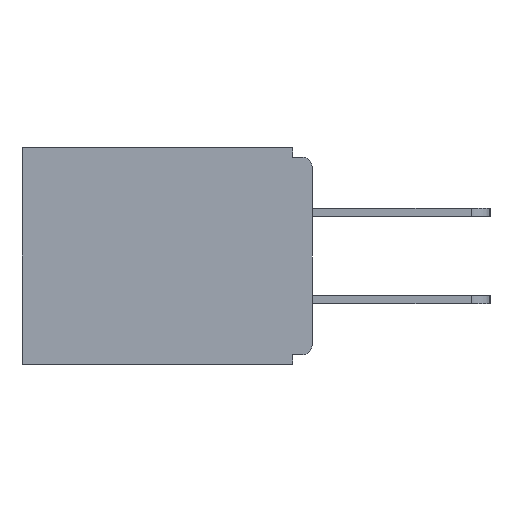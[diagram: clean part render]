
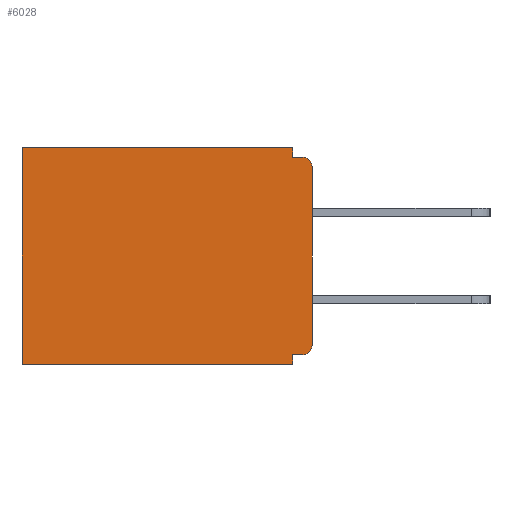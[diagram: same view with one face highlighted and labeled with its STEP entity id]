
A CAD part, left-side view. The second image highlights one B-rep face of the part: STEP entity #6028.
In plain terms, the highlighted planar face has unit normal (-1, 0, 0).
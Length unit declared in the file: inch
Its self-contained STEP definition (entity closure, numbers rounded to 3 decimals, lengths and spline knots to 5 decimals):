
#11 = DIRECTION ( 'NONE',  ( 0., 1., 0. ) ) ;
#64 = FACE_OUTER_BOUND ( 'NONE', #15069, .T. ) ;
#215 = CARTESIAN_POINT ( 'NONE',  ( 0.298, 0., 0. ) ) ;
#602 = CARTESIAN_POINT ( 'NONE',  ( 0.298, 0.46, 0. ) ) ;
#608 = CARTESIAN_POINT ( 'NONE',  ( 0.298, 0.015, -0.03 ) ) ;
#649 = EDGE_CURVE ( 'NONE', #14094, #7322, #11745, .T. ) ;
#720 = VERTEX_POINT ( 'NONE', #4640 ) ;
#843 = CARTESIAN_POINT ( 'NONE',  ( 0.298, 0.031, -0.328 ) ) ;
#852 = EDGE_CURVE ( 'NONE', #11804, #15190, #6631, .T. ) ;
#913 = CIRCLE ( 'NONE', #3900, 0.015 ) ;
#1393 = CARTESIAN_POINT ( 'NONE',  ( 0.298, 0., -0.328 ) ) ;
#1752 = DIRECTION ( 'NONE',  ( 0., 0., -1. ) ) ;
#1772 = EDGE_CURVE ( 'NONE', #8749, #11788, #9150, .T. ) ;
#1929 = EDGE_CURVE ( 'NONE', #8749, #8089, #913, .T. ) ;
#2043 = CARTESIAN_POINT ( 'NONE',  ( 0.298, 0., -0.03 ) ) ;
#2549 = VECTOR ( 'NONE', #9634, 39.37008 ) ;
#2890 = DIRECTION ( 'NONE',  ( -1., 0., 0. ) ) ;
#3313 = EDGE_CURVE ( 'NONE', #720, #7322, #11913, .T. ) ;
#3400 = CIRCLE ( 'NONE', #14229, 0.015 ) ;
#3420 = LINE ( 'NONE', #4873, #13512 ) ;
#3453 = VECTOR ( 'NONE', #11, 39.37008 ) ;
#3592 = ORIENTED_EDGE ( 'NONE', *, *, #13378, .F. ) ;
#3638 = CARTESIAN_POINT ( 'NONE',  ( 0.298, 0., 0. ) ) ;
#3900 = AXIS2_PLACEMENT_3D ( 'NONE', #5189, #10061, #6422 ) ;
#3957 = LINE ( 'NONE', #6035, #8710 ) ;
#4184 = DIRECTION ( 'NONE',  ( 0., 0., -1. ) ) ;
#4640 = CARTESIAN_POINT ( 'NONE',  ( 0.298, 0.031, -0.343 ) ) ;
#4873 = CARTESIAN_POINT ( 'NONE',  ( 0.298, 0., -0.015 ) ) ;
#4896 = ORIENTED_EDGE ( 'NONE', *, *, #852, .F. ) ;
#4898 = PLANE ( 'NONE',  #9255 ) ;
#5189 = CARTESIAN_POINT ( 'NONE',  ( 0.298, 0.015, -0.313 ) ) ;
#5520 = EDGE_CURVE ( 'NONE', #7684, #11739, #3400, .T. ) ;
#5567 = CARTESIAN_POINT ( 'NONE',  ( 0.298, 0., 0. ) ) ;
#5697 = ORIENTED_EDGE ( 'NONE', *, *, #1772, .F. ) ;
#5848 = ORIENTED_EDGE ( 'NONE', *, *, #5520, .T. ) ;
#6028 = ADVANCED_FACE ( 'NONE', ( #64 ), #4898, .F. ) ;
#6035 = CARTESIAN_POINT ( 'NONE',  ( 0.298, 0.031, -0.343 ) ) ;
#6422 = DIRECTION ( 'NONE',  ( 0., 0., -1. ) ) ;
#6631 = LINE ( 'NONE', #11407, #13027 ) ;
#6673 = EDGE_CURVE ( 'NONE', #11804, #14094, #13453, .T. ) ;
#7056 = VECTOR ( 'NONE', #9586, 39.37008 ) ;
#7313 = CARTESIAN_POINT ( 'NONE',  ( 0.298, 0.031, -0.015 ) ) ;
#7322 = VERTEX_POINT ( 'NONE', #14557 ) ;
#7684 = VERTEX_POINT ( 'NONE', #2043 ) ;
#8089 = VERTEX_POINT ( 'NONE', #11778 ) ;
#8325 = ORIENTED_EDGE ( 'NONE', *, *, #6673, .T. ) ;
#8421 = ORIENTED_EDGE ( 'NONE', *, *, #1929, .T. ) ;
#8512 = DIRECTION ( 'NONE',  ( 0., -1., 0. ) ) ;
#8710 = VECTOR ( 'NONE', #13284, 39.37008 ) ;
#8749 = VERTEX_POINT ( 'NONE', #12000 ) ;
#8943 = VECTOR ( 'NONE', #4184, 39.37008 ) ;
#9150 = LINE ( 'NONE', #1393, #2549 ) ;
#9255 = AXIS2_PLACEMENT_3D ( 'NONE', #215, #14837, #1752 ) ;
#9586 = DIRECTION ( 'NONE',  ( 0., 0., -1. ) ) ;
#9634 = DIRECTION ( 'NONE',  ( 0., 1., 0. ) ) ;
#10061 = DIRECTION ( 'NONE',  ( -1., 0., 0. ) ) ;
#10394 = ORIENTED_EDGE ( 'NONE', *, *, #13157, .F. ) ;
#10799 = CARTESIAN_POINT ( 'NONE',  ( 0.298, 0.015, -0.015 ) ) ;
#11304 = DIRECTION ( 'NONE',  ( 0., 0., -1. ) ) ;
#11407 = CARTESIAN_POINT ( 'NONE',  ( 0.298, 0.031, -0.343 ) ) ;
#11495 = CARTESIAN_POINT ( 'NONE',  ( 0.298, 0.46, 0. ) ) ;
#11739 = VERTEX_POINT ( 'NONE', #10799 ) ;
#11745 = LINE ( 'NONE', #11495, #7056 ) ;
#11769 = LINE ( 'NONE', #5567, #8943 ) ;
#11778 = CARTESIAN_POINT ( 'NONE',  ( 0.298, 0., -0.313 ) ) ;
#11788 = VERTEX_POINT ( 'NONE', #843 ) ;
#11804 = VERTEX_POINT ( 'NONE', #12728 ) ;
#11913 = LINE ( 'NONE', #14531, #3453 ) ;
#12000 = CARTESIAN_POINT ( 'NONE',  ( 0.298, 0.015, -0.328 ) ) ;
#12728 = CARTESIAN_POINT ( 'NONE',  ( 0.298, 0.031, 0. ) ) ;
#13027 = VECTOR ( 'NONE', #11304, 39.37008 ) ;
#13065 = EDGE_CURVE ( 'NONE', #15190, #11739, #3420, .T. ) ;
#13157 = EDGE_CURVE ( 'NONE', #11788, #720, #3957, .T. ) ;
#13201 = DIRECTION ( 'NONE',  ( 0., 1., 0. ) ) ;
#13284 = DIRECTION ( 'NONE',  ( 0., 0., -1. ) ) ;
#13378 = EDGE_CURVE ( 'NONE', #7684, #8089, #11769, .T. ) ;
#13453 = LINE ( 'NONE', #3638, #14580 ) ;
#13512 = VECTOR ( 'NONE', #8512, 39.37008 ) ;
#14074 = ORIENTED_EDGE ( 'NONE', *, *, #649, .T. ) ;
#14094 = VERTEX_POINT ( 'NONE', #602 ) ;
#14229 = AXIS2_PLACEMENT_3D ( 'NONE', #608, #2890, #14731 ) ;
#14531 = CARTESIAN_POINT ( 'NONE',  ( 0.298, 0., -0.343 ) ) ;
#14557 = CARTESIAN_POINT ( 'NONE',  ( 0.298, 0.46, -0.343 ) ) ;
#14580 = VECTOR ( 'NONE', #13201, 39.37008 ) ;
#14731 = DIRECTION ( 'NONE',  ( 0., 0., -1. ) ) ;
#14755 = ORIENTED_EDGE ( 'NONE', *, *, #3313, .F. ) ;
#14837 = DIRECTION ( 'NONE',  ( 1., 0., 0. ) ) ;
#15069 = EDGE_LOOP ( 'NONE', ( #5848, #15246, #4896, #8325, #14074, #14755, #10394, #5697, #8421, #3592 ) ) ;
#15190 = VERTEX_POINT ( 'NONE', #7313 ) ;
#15246 = ORIENTED_EDGE ( 'NONE', *, *, #13065, .F. ) ;
